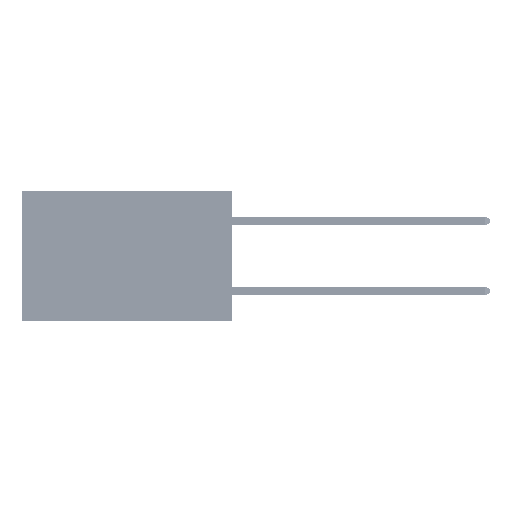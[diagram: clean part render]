
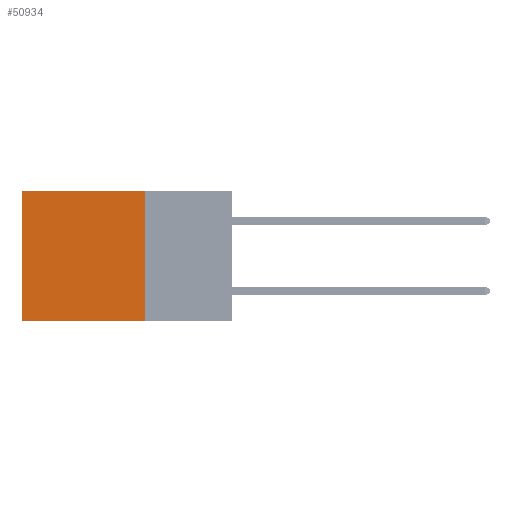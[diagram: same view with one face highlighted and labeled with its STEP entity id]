
A CAD part, left-side view. The second image highlights one B-rep face of the part: STEP entity #50934.
In plain terms, the highlighted planar face has unit normal (-1, 0, 0).
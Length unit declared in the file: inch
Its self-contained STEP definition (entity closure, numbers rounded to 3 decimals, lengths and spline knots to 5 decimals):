
#1912 = ORIENTED_EDGE ( 'NONE', *, *, #42911, .T. ) ;
#4491 = VERTEX_POINT ( 'NONE', #26553 ) ;
#4590 = VERTEX_POINT ( 'NONE', #11233 ) ;
#4916 = LINE ( 'NONE', #40275, #21294 ) ;
#5419 = VERTEX_POINT ( 'NONE', #15916 ) ;
#6583 = DIRECTION ( 'NONE',  ( 0., 0., -1. ) ) ;
#8052 = EDGE_CURVE ( 'NONE', #5419, #4491, #4916, .T. ) ;
#11233 = CARTESIAN_POINT ( 'NONE',  ( 0.2875, 0.25, 0. ) ) ;
#12680 = DIRECTION ( 'NONE',  ( 1., 0., 0. ) ) ;
#15916 = CARTESIAN_POINT ( 'NONE',  ( 0.2875, 0.25, -0.37 ) ) ;
#17083 = DIRECTION ( 'NONE',  ( 0., 0., -1. ) ) ;
#20612 = DIRECTION ( 'NONE',  ( 0., 0., -1. ) ) ;
#21294 = VECTOR ( 'NONE', #48402, 39.37008 ) ;
#21451 = CARTESIAN_POINT ( 'NONE',  ( 0.2875, 0.25, 0. ) ) ;
#23046 = AXIS2_PLACEMENT_3D ( 'NONE', #33471, #12680, #17083 ) ;
#23784 = ORIENTED_EDGE ( 'NONE', *, *, #8052, .F. ) ;
#26553 = CARTESIAN_POINT ( 'NONE',  ( 0.2875, 0.6, -0.37 ) ) ;
#26594 = ORIENTED_EDGE ( 'NONE', *, *, #44670, .T. ) ;
#26820 = FACE_OUTER_BOUND ( 'NONE', #50502, .T. ) ;
#29584 = VERTEX_POINT ( 'NONE', #42667 ) ;
#31139 = VECTOR ( 'NONE', #49709, 39.37008 ) ;
#33471 = CARTESIAN_POINT ( 'NONE',  ( 0.2875, 0.25, 0. ) ) ;
#37154 = VECTOR ( 'NONE', #20612, 39.37008 ) ;
#38501 = CARTESIAN_POINT ( 'NONE',  ( 0.2875, 0.25, 0. ) ) ;
#40275 = CARTESIAN_POINT ( 'NONE',  ( 0.2875, 0.25, -0.37 ) ) ;
#40466 = LINE ( 'NONE', #38501, #48691 ) ;
#41273 = PLANE ( 'NONE',  #23046 ) ;
#41927 = ORIENTED_EDGE ( 'NONE', *, *, #49768, .F. ) ;
#42667 = CARTESIAN_POINT ( 'NONE',  ( 0.2875, 0.6, 0. ) ) ;
#42911 = EDGE_CURVE ( 'NONE', #4590, #29584, #51370, .T. ) ;
#43501 = LINE ( 'NONE', #48165, #37154 ) ;
#44670 = EDGE_CURVE ( 'NONE', #29584, #4491, #43501, .T. ) ;
#48165 = CARTESIAN_POINT ( 'NONE',  ( 0.2875, 0.6, 0. ) ) ;
#48402 = DIRECTION ( 'NONE',  ( 0., 1., 0. ) ) ;
#48691 = VECTOR ( 'NONE', #6583, 39.37008 ) ;
#49709 = DIRECTION ( 'NONE',  ( 0., 1., 0. ) ) ;
#49768 = EDGE_CURVE ( 'NONE', #4590, #5419, #40466, .T. ) ;
#50502 = EDGE_LOOP ( 'NONE', ( #26594, #23784, #41927, #1912 ) ) ;
#50934 = ADVANCED_FACE ( 'NONE', ( #26820 ), #41273, .F. ) ;
#51370 = LINE ( 'NONE', #21451, #31139 ) ;
